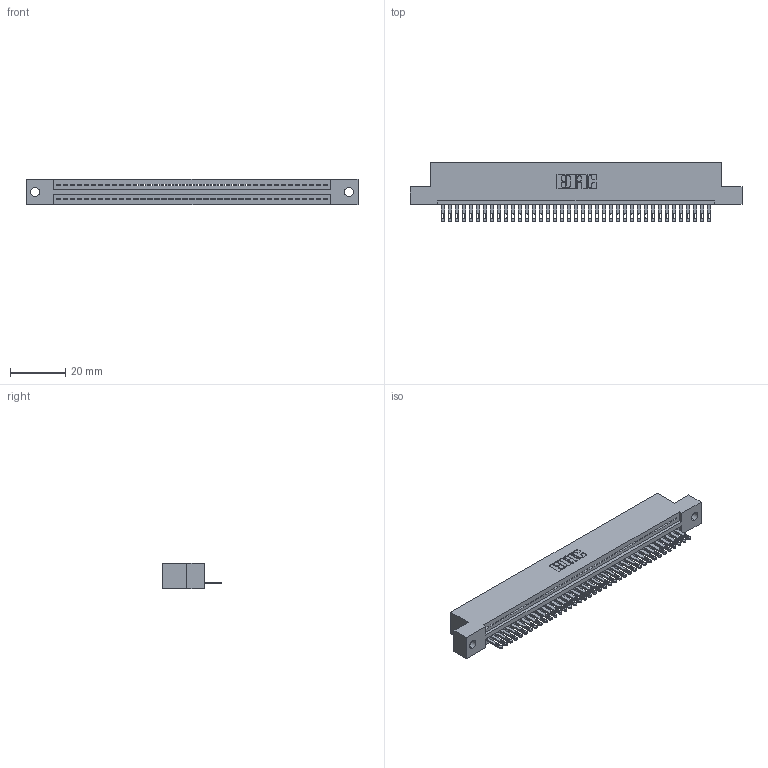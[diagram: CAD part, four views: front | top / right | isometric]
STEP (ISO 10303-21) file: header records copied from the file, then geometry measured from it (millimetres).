
FILE_DESCRIPTION (( 'STEP AP203' ), '1' );
FILE_NAME ('345-039-500-102.STEP', '2019-10-08T05:07:32', ( '' ), ( '' ), 'SwSTEP 2.0', 'SolidWorks 2016', '' );
FILE_SCHEMA (( 'CONFIG_CONTROL_DESIGN' ));
Length unit declared in the file: inch
Products named in the file (3): 345-039-500-102; 345-292-001_345-293-100; 345 Part_Flush Mounting Lugs - 0.128 Dia
Assembly tree (40 placements, depth 2):
  345-039-500-102
    345 Part_Flush Mounting Lugs - 0.128 Dia
    345-292-001_345-293-100  x39
Bounding box: 120.27 x 21.51 x 9.4 mm (x, y, z)
Volume: 11386.2 mm3; surface area: 14906.5 mm2
Topology: 40 solids, 40 shells, 2232 faces, 6893 edges, 4594 vertices
Faces by surface type: plane 1406, cylinder 826
Entity records: 29689 total; most frequent: CARTESIAN_POINT 5149, ORIENTED_EDGE 5122, DIRECTION 4503, EDGE_CURVE 2561, VECTOR 2269, LINE 2269, VERTEX_POINT 1706, AXIS2_PLACEMENT_3D 1117
